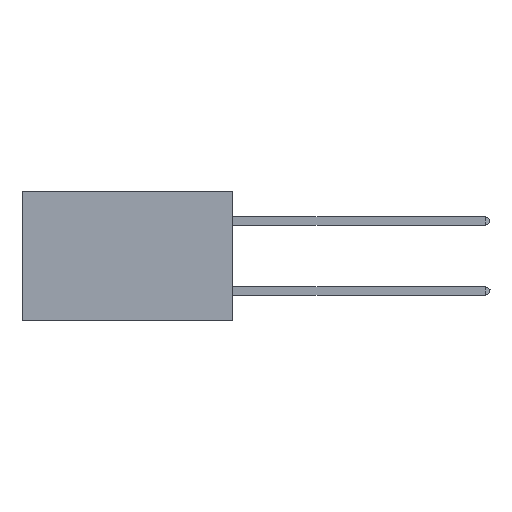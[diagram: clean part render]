
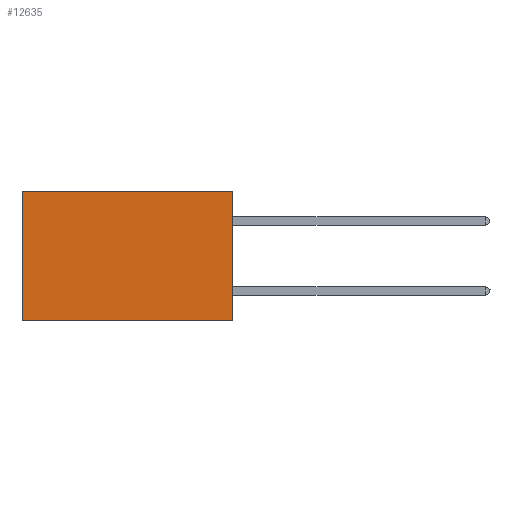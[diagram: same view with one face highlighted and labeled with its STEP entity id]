
A CAD part, left-side view. The second image highlights one B-rep face of the part: STEP entity #12635.
In plain terms, the highlighted planar face has unit normal (-1, 0, 0).
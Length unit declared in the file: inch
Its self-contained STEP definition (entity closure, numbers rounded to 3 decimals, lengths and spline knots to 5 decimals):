
#387 = EDGE_CURVE ( 'NONE', #1075, #14599, #1112, .T. ) ;
#661 = VECTOR ( 'NONE', #3658, 39.37008 ) ;
#1075 = VERTEX_POINT ( 'NONE', #3422 ) ;
#1112 = LINE ( 'NONE', #5728, #661 ) ;
#1240 = DIRECTION ( 'NONE',  ( 0., 1., 0. ) ) ;
#1679 = ORIENTED_EDGE ( 'NONE', *, *, #387, .F. ) ;
#1889 = VECTOR ( 'NONE', #2155, 39.37008 ) ;
#2155 = DIRECTION ( 'NONE',  ( 0., 0., -1. ) ) ;
#2350 = CARTESIAN_POINT ( 'NONE',  ( 0.2875, 0., 0. ) ) ;
#2611 = ORIENTED_EDGE ( 'NONE', *, *, #6523, .T. ) ;
#3416 = CARTESIAN_POINT ( 'NONE',  ( 0.2875, 0.6, 0. ) ) ;
#3422 = CARTESIAN_POINT ( 'NONE',  ( 0.2875, 0., -0.37 ) ) ;
#3658 = DIRECTION ( 'NONE',  ( 0., 1., 0. ) ) ;
#5547 = LINE ( 'NONE', #7488, #8321 ) ;
#5728 = CARTESIAN_POINT ( 'NONE',  ( 0.2875, 0., -0.37 ) ) ;
#5730 = PLANE ( 'NONE',  #12825 ) ;
#6523 = EDGE_CURVE ( 'NONE', #16436, #14293, #7025, .T. ) ;
#7025 = LINE ( 'NONE', #2350, #14258 ) ;
#7115 = DIRECTION ( 'NONE',  ( 1., 0., 0. ) ) ;
#7488 = CARTESIAN_POINT ( 'NONE',  ( 0.2875, 0., 0. ) ) ;
#8147 = EDGE_LOOP ( 'NONE', ( #15349, #1679, #9053, #2611 ) ) ;
#8203 = CARTESIAN_POINT ( 'NONE',  ( 0.2875, 0., 0. ) ) ;
#8321 = VECTOR ( 'NONE', #15101, 39.37008 ) ;
#8723 = FACE_OUTER_BOUND ( 'NONE', #8147, .T. ) ;
#9053 = ORIENTED_EDGE ( 'NONE', *, *, #12223, .F. ) ;
#9437 = EDGE_CURVE ( 'NONE', #14293, #14599, #12627, .T. ) ;
#9728 = CARTESIAN_POINT ( 'NONE',  ( 0.2875, 0., 0. ) ) ;
#10331 = CARTESIAN_POINT ( 'NONE',  ( 0.2875, 0.6, 0. ) ) ;
#12223 = EDGE_CURVE ( 'NONE', #16436, #1075, #5547, .T. ) ;
#12627 = LINE ( 'NONE', #10331, #1889 ) ;
#12635 = ADVANCED_FACE ( 'NONE', ( #8723 ), #5730, .F. ) ;
#12825 = AXIS2_PLACEMENT_3D ( 'NONE', #9728, #7115, #16016 ) ;
#14258 = VECTOR ( 'NONE', #1240, 39.37008 ) ;
#14293 = VERTEX_POINT ( 'NONE', #3416 ) ;
#14599 = VERTEX_POINT ( 'NONE', #15831 ) ;
#15101 = DIRECTION ( 'NONE',  ( 0., 0., -1. ) ) ;
#15349 = ORIENTED_EDGE ( 'NONE', *, *, #9437, .T. ) ;
#15831 = CARTESIAN_POINT ( 'NONE',  ( 0.2875, 0.6, -0.37 ) ) ;
#16016 = DIRECTION ( 'NONE',  ( 0., 0., -1. ) ) ;
#16436 = VERTEX_POINT ( 'NONE', #8203 ) ;
